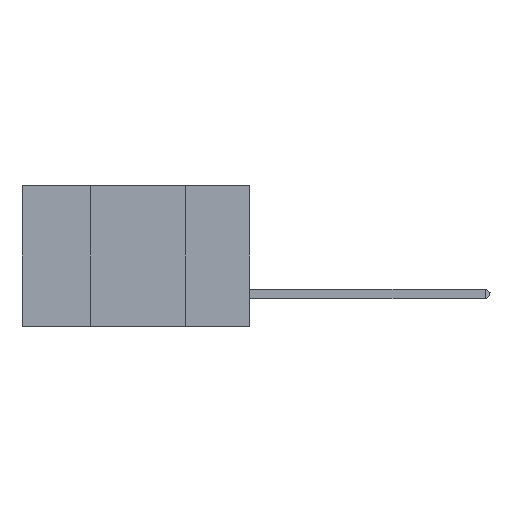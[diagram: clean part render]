
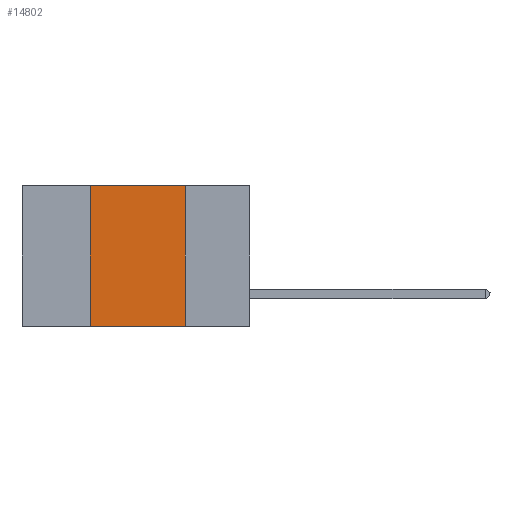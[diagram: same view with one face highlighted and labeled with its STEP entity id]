
A CAD part, left-side view. The second image highlights one B-rep face of the part: STEP entity #14802.
In plain terms, the highlighted planar face has unit normal (-1, 0, 0).
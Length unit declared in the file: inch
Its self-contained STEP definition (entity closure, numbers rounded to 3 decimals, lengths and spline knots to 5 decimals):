
#2985 = ORIENTED_EDGE ( 'NONE', *, *, #42888, .F. ) ;
#3655 = EDGE_LOOP ( 'NONE', ( #28425, #2985, #21516, #24071 ) ) ;
#3831 = LINE ( 'NONE', #32802, #39620 ) ;
#4518 = VERTEX_POINT ( 'NONE', #30665 ) ;
#6566 = CARTESIAN_POINT ( 'NONE',  ( 0., 0.42, -0.37 ) ) ;
#6753 = LINE ( 'NONE', #43443, #40922 ) ;
#8217 = CARTESIAN_POINT ( 'NONE',  ( 0., 0.42, 0. ) ) ;
#9312 = CARTESIAN_POINT ( 'NONE',  ( 0., 0.17, -0.37 ) ) ;
#10110 = AXIS2_PLACEMENT_3D ( 'NONE', #21384, #11124, #34976 ) ;
#11124 = DIRECTION ( 'NONE',  ( 1., 0., 0. ) ) ;
#14802 = ADVANCED_FACE ( 'NONE', ( #35191 ), #41674, .F. ) ;
#15787 = DIRECTION ( 'NONE',  ( 0., 0., -1. ) ) ;
#16742 = DIRECTION ( 'NONE',  ( 0., -1., 0. ) ) ;
#18185 = EDGE_CURVE ( 'NONE', #33452, #39352, #3831, .T. ) ;
#18536 = DIRECTION ( 'NONE',  ( 0., 0., 1. ) ) ;
#21324 = LINE ( 'NONE', #8217, #41620 ) ;
#21384 = CARTESIAN_POINT ( 'NONE',  ( 0., 0.6, 0. ) ) ;
#21516 = ORIENTED_EDGE ( 'NONE', *, *, #21935, .F. ) ;
#21750 = CARTESIAN_POINT ( 'NONE',  ( 0., 0.17, 0. ) ) ;
#21935 = EDGE_CURVE ( 'NONE', #29692, #4518, #21324, .T. ) ;
#22649 = EDGE_CURVE ( 'NONE', #29692, #39352, #30904, .T. ) ;
#24071 = ORIENTED_EDGE ( 'NONE', *, *, #22649, .T. ) ;
#28425 = ORIENTED_EDGE ( 'NONE', *, *, #18185, .F. ) ;
#29692 = VERTEX_POINT ( 'NONE', #6566 ) ;
#30665 = CARTESIAN_POINT ( 'NONE',  ( 0., 0.42, 0. ) ) ;
#30904 = LINE ( 'NONE', #34092, #43232 ) ;
#32802 = CARTESIAN_POINT ( 'NONE',  ( 0., 0.17, 0. ) ) ;
#33452 = VERTEX_POINT ( 'NONE', #21750 ) ;
#33675 = DIRECTION ( 'NONE',  ( 0., -1., 0. ) ) ;
#34092 = CARTESIAN_POINT ( 'NONE',  ( 0., 0.6, -0.37 ) ) ;
#34976 = DIRECTION ( 'NONE',  ( 0., 0., -1. ) ) ;
#35191 = FACE_OUTER_BOUND ( 'NONE', #3655, .T. ) ;
#39352 = VERTEX_POINT ( 'NONE', #9312 ) ;
#39620 = VECTOR ( 'NONE', #15787, 39.37008 ) ;
#40922 = VECTOR ( 'NONE', #16742, 39.37008 ) ;
#41620 = VECTOR ( 'NONE', #18536, 39.37008 ) ;
#41674 = PLANE ( 'NONE',  #10110 ) ;
#42888 = EDGE_CURVE ( 'NONE', #4518, #33452, #6753, .T. ) ;
#43232 = VECTOR ( 'NONE', #33675, 39.37008 ) ;
#43443 = CARTESIAN_POINT ( 'NONE',  ( 0., 0.6, 0. ) ) ;
